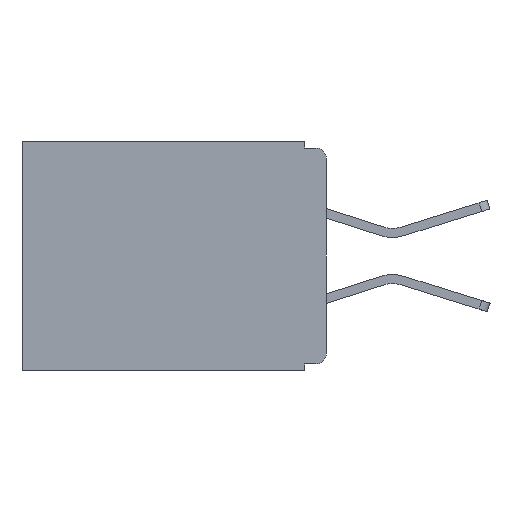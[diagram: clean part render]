
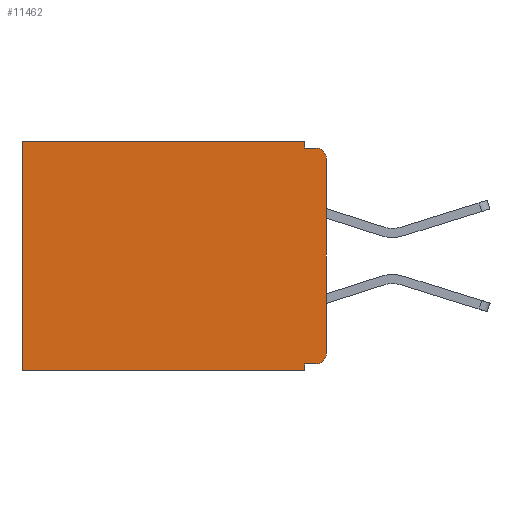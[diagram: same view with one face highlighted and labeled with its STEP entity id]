
A CAD part, left-side view. The second image highlights one B-rep face of the part: STEP entity #11462.
In plain terms, the highlighted planar face has unit normal (-1, 0, 0).
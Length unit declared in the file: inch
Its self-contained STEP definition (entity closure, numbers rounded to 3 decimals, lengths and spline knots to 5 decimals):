
#182 = EDGE_CURVE ( 'NONE', #11762, #6344, #4981, .T. ) ;
#227 = DIRECTION ( 'NONE',  ( 0., 0., -1. ) ) ;
#771 = DIRECTION ( 'NONE',  ( -1., 0., 0. ) ) ;
#1025 = LINE ( 'NONE', #11363, #7350 ) ;
#1150 = EDGE_CURVE ( 'NONE', #9400, #5718, #14663, .T. ) ;
#1817 = VECTOR ( 'NONE', #10985, 39.37008 ) ;
#1908 = VECTOR ( 'NONE', #12636, 39.37008 ) ;
#2025 = ORIENTED_EDGE ( 'NONE', *, *, #5527, .T. ) ;
#2054 = CARTESIAN_POINT ( 'NONE',  ( 0.3, 0., -0.305 ) ) ;
#2385 = AXIS2_PLACEMENT_3D ( 'NONE', #15249, #7870, #227 ) ;
#2629 = VERTEX_POINT ( 'NONE', #4982 ) ;
#2927 = AXIS2_PLACEMENT_3D ( 'NONE', #8405, #771, #9680 ) ;
#3129 = ORIENTED_EDGE ( 'NONE', *, *, #182, .F. ) ;
#3364 = EDGE_CURVE ( 'NONE', #6344, #14146, #14044, .T. ) ;
#3657 = VECTOR ( 'NONE', #12386, 39.37008 ) ;
#3781 = CARTESIAN_POINT ( 'NONE',  ( 0.3, 0., -0.01 ) ) ;
#3879 = CARTESIAN_POINT ( 'NONE',  ( 0.3, 0.015, -0.01 ) ) ;
#4981 = LINE ( 'NONE', #9452, #13731 ) ;
#4982 = CARTESIAN_POINT ( 'NONE',  ( 0.3, 0.015, -0.32 ) ) ;
#5060 = CARTESIAN_POINT ( 'NONE',  ( 0.3, 0.031, -0.32 ) ) ;
#5093 = ORIENTED_EDGE ( 'NONE', *, *, #3364, .F. ) ;
#5246 = LINE ( 'NONE', #8914, #1908 ) ;
#5431 = CARTESIAN_POINT ( 'NONE',  ( 0.3, 0., -0.33 ) ) ;
#5465 = VECTOR ( 'NONE', #11525, 39.37008 ) ;
#5527 = EDGE_CURVE ( 'NONE', #9126, #12915, #1025, .T. ) ;
#5718 = VERTEX_POINT ( 'NONE', #15454 ) ;
#5978 = EDGE_CURVE ( 'NONE', #2629, #9400, #14319, .T. ) ;
#6130 = EDGE_LOOP ( 'NONE', ( #8657, #15333, #5093, #3129, #14027, #2025, #15745, #14299, #8836, #11035 ) ) ;
#6344 = VERTEX_POINT ( 'NONE', #15368 ) ;
#6353 = CIRCLE ( 'NONE', #2385, 0.015 ) ;
#6680 = DIRECTION ( 'NONE',  ( 1., 0., 0. ) ) ;
#7184 = AXIS2_PLACEMENT_3D ( 'NONE', #5431, #6680, #15321 ) ;
#7338 = VECTOR ( 'NONE', #7391, 39.37008 ) ;
#7350 = VECTOR ( 'NONE', #12709, 39.37008 ) ;
#7360 = CARTESIAN_POINT ( 'NONE',  ( 0.3, 0.437, 0. ) ) ;
#7391 = DIRECTION ( 'NONE',  ( 0., 1., 0. ) ) ;
#7399 = FACE_OUTER_BOUND ( 'NONE', #6130, .T. ) ;
#7870 = DIRECTION ( 'NONE',  ( -1., 0., 0. ) ) ;
#8140 = DIRECTION ( 'NONE',  ( 0., -1., 0. ) ) ;
#8405 = CARTESIAN_POINT ( 'NONE',  ( 0.3, 0.015, -0.025 ) ) ;
#8657 = ORIENTED_EDGE ( 'NONE', *, *, #15403, .F. ) ;
#8836 = ORIENTED_EDGE ( 'NONE', *, *, #5978, .F. ) ;
#8914 = CARTESIAN_POINT ( 'NONE',  ( 0.3, 0., -0.33 ) ) ;
#9126 = VERTEX_POINT ( 'NONE', #7360 ) ;
#9400 = VERTEX_POINT ( 'NONE', #5060 ) ;
#9452 = CARTESIAN_POINT ( 'NONE',  ( 0.3, 0.031, 0. ) ) ;
#9680 = DIRECTION ( 'NONE',  ( 0., 0., -1. ) ) ;
#9756 = VERTEX_POINT ( 'NONE', #2054 ) ;
#10225 = CARTESIAN_POINT ( 'NONE',  ( 0.3, 0., -0.33 ) ) ;
#10354 = LINE ( 'NONE', #11165, #3657 ) ;
#10697 = EDGE_CURVE ( 'NONE', #5718, #12915, #12523, .T. ) ;
#10985 = DIRECTION ( 'NONE',  ( 0., 0., -1. ) ) ;
#11035 = ORIENTED_EDGE ( 'NONE', *, *, #13670, .T. ) ;
#11165 = CARTESIAN_POINT ( 'NONE',  ( 0.3, 0., 0. ) ) ;
#11199 = VECTOR ( 'NONE', #8140, 39.37008 ) ;
#11363 = CARTESIAN_POINT ( 'NONE',  ( 0.3, 0.437, -0.33 ) ) ;
#11462 = ADVANCED_FACE ( 'NONE', ( #7399 ), #12914, .F. ) ;
#11525 = DIRECTION ( 'NONE',  ( 0., 1., 0. ) ) ;
#11762 = VERTEX_POINT ( 'NONE', #15900 ) ;
#11801 = CARTESIAN_POINT ( 'NONE',  ( 0.3, 0., -0.025 ) ) ;
#12119 = VERTEX_POINT ( 'NONE', #11801 ) ;
#12386 = DIRECTION ( 'NONE',  ( 0., 1., 0. ) ) ;
#12523 = LINE ( 'NONE', #10225, #5465 ) ;
#12636 = DIRECTION ( 'NONE',  ( 0., 0., -1. ) ) ;
#12709 = DIRECTION ( 'NONE',  ( 0., 0., -1. ) ) ;
#12914 = PLANE ( 'NONE',  #7184 ) ;
#12915 = VERTEX_POINT ( 'NONE', #15969 ) ;
#13402 = EDGE_CURVE ( 'NONE', #11762, #9126, #10354, .T. ) ;
#13670 = EDGE_CURVE ( 'NONE', #2629, #9756, #6353, .T. ) ;
#13731 = VECTOR ( 'NONE', #15680, 39.37008 ) ;
#13879 = EDGE_CURVE ( 'NONE', #12119, #14146, #16000, .T. ) ;
#14027 = ORIENTED_EDGE ( 'NONE', *, *, #13402, .T. ) ;
#14044 = LINE ( 'NONE', #3781, #11199 ) ;
#14146 = VERTEX_POINT ( 'NONE', #3879 ) ;
#14295 = CARTESIAN_POINT ( 'NONE',  ( 0.3, 0.031, -0.33 ) ) ;
#14299 = ORIENTED_EDGE ( 'NONE', *, *, #1150, .F. ) ;
#14319 = LINE ( 'NONE', #16221, #7338 ) ;
#14663 = LINE ( 'NONE', #14295, #1817 ) ;
#15249 = CARTESIAN_POINT ( 'NONE',  ( 0.3, 0.015, -0.305 ) ) ;
#15321 = DIRECTION ( 'NONE',  ( 0., 0., -1. ) ) ;
#15333 = ORIENTED_EDGE ( 'NONE', *, *, #13879, .T. ) ;
#15368 = CARTESIAN_POINT ( 'NONE',  ( 0.3, 0.031, -0.01 ) ) ;
#15403 = EDGE_CURVE ( 'NONE', #12119, #9756, #5246, .T. ) ;
#15454 = CARTESIAN_POINT ( 'NONE',  ( 0.3, 0.031, -0.33 ) ) ;
#15680 = DIRECTION ( 'NONE',  ( 0., 0., -1. ) ) ;
#15745 = ORIENTED_EDGE ( 'NONE', *, *, #10697, .F. ) ;
#15900 = CARTESIAN_POINT ( 'NONE',  ( 0.3, 0.031, 0. ) ) ;
#15969 = CARTESIAN_POINT ( 'NONE',  ( 0.3, 0.437, -0.33 ) ) ;
#16000 = CIRCLE ( 'NONE', #2927, 0.015 ) ;
#16221 = CARTESIAN_POINT ( 'NONE',  ( 0.3, 0., -0.32 ) ) ;
